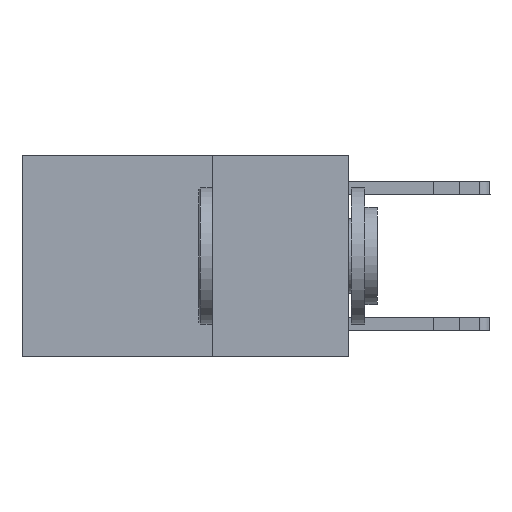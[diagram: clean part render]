
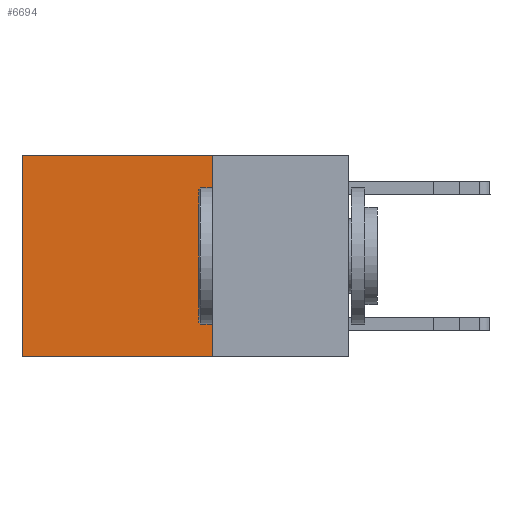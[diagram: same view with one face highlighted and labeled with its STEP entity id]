
A CAD part, left-side view. The second image highlights one B-rep face of the part: STEP entity #6694.
In plain terms, the highlighted planar face has unit normal (-1, 0, 0).
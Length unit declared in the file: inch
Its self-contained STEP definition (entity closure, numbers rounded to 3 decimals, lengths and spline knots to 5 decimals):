
#680 = PLANE ( 'NONE',  #1129 ) ;
#1129 = AXIS2_PLACEMENT_3D ( 'NONE', #10428, #20315, #8923 ) ;
#1700 = LINE ( 'NONE', #19842, #19647 ) ;
#3120 = EDGE_CURVE ( 'NONE', #13688, #15120, #16413, .T. ) ;
#3169 = DIRECTION ( 'NONE',  ( 0., 0., -1. ) ) ;
#3791 = VERTEX_POINT ( 'NONE', #6617 ) ;
#4253 = ORIENTED_EDGE ( 'NONE', *, *, #3120, .T. ) ;
#4767 = ORIENTED_EDGE ( 'NONE', *, *, #5166, .F. ) ;
#5166 = EDGE_CURVE ( 'NONE', #3791, #8269, #15022, .T. ) ;
#6617 = CARTESIAN_POINT ( 'NONE',  ( 0.2625, 0.25, 0. ) ) ;
#6694 = ADVANCED_FACE ( 'NONE', ( #8710 ), #680, .F. ) ;
#7741 = CARTESIAN_POINT ( 'NONE',  ( 0.2625, 0.25, -0.37 ) ) ;
#8269 = VERTEX_POINT ( 'NONE', #7741 ) ;
#8710 = FACE_OUTER_BOUND ( 'NONE', #17575, .T. ) ;
#8923 = DIRECTION ( 'NONE',  ( 0., 0., -1. ) ) ;
#10428 = CARTESIAN_POINT ( 'NONE',  ( 0.2625, 0.25, 0. ) ) ;
#10976 = EDGE_CURVE ( 'NONE', #8269, #15120, #1700, .T. ) ;
#11179 = LINE ( 'NONE', #17955, #14580 ) ;
#11571 = DIRECTION ( 'NONE',  ( 0., 1., 0. ) ) ;
#12110 = ORIENTED_EDGE ( 'NONE', *, *, #12372, .T. ) ;
#12205 = CARTESIAN_POINT ( 'NONE',  ( 0.2625, 0.6, -0.37 ) ) ;
#12372 = EDGE_CURVE ( 'NONE', #3791, #13688, #11179, .T. ) ;
#12698 = DIRECTION ( 'NONE',  ( 0., 1., 0. ) ) ;
#13688 = VERTEX_POINT ( 'NONE', #14111 ) ;
#13966 = VECTOR ( 'NONE', #3169, 39.37008 ) ;
#14111 = CARTESIAN_POINT ( 'NONE',  ( 0.2625, 0.6, 0. ) ) ;
#14580 = VECTOR ( 'NONE', #12698, 39.37008 ) ;
#15022 = LINE ( 'NONE', #18530, #15519 ) ;
#15120 = VERTEX_POINT ( 'NONE', #12205 ) ;
#15222 = DIRECTION ( 'NONE',  ( 0., 0., -1. ) ) ;
#15519 = VECTOR ( 'NONE', #15222, 39.37008 ) ;
#16413 = LINE ( 'NONE', #19504, #13966 ) ;
#17392 = ORIENTED_EDGE ( 'NONE', *, *, #10976, .F. ) ;
#17575 = EDGE_LOOP ( 'NONE', ( #4253, #17392, #4767, #12110 ) ) ;
#17955 = CARTESIAN_POINT ( 'NONE',  ( 0.2625, 0.25, 0. ) ) ;
#18530 = CARTESIAN_POINT ( 'NONE',  ( 0.2625, 0.25, 0. ) ) ;
#19504 = CARTESIAN_POINT ( 'NONE',  ( 0.2625, 0.6, 0. ) ) ;
#19647 = VECTOR ( 'NONE', #11571, 39.37008 ) ;
#19842 = CARTESIAN_POINT ( 'NONE',  ( 0.2625, 0.25, -0.37 ) ) ;
#20315 = DIRECTION ( 'NONE',  ( 1., 0., 0. ) ) ;
